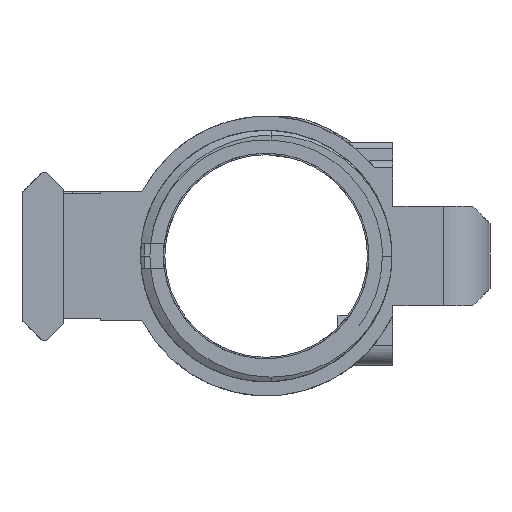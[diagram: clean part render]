
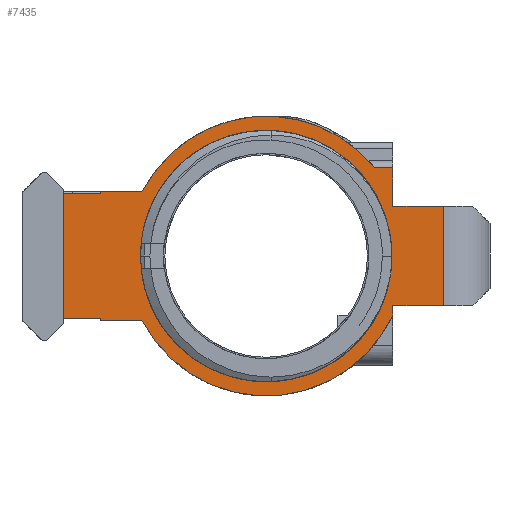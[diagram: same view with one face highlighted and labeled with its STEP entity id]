
A CAD part, left-side view. The second image highlights one B-rep face of the part: STEP entity #7435.
In plain terms, the highlighted planar face has unit normal (-1, 0, 0).
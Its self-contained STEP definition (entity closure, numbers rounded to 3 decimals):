
#105=FACE_BOUND('',#1064,.T.);
#117=CIRCLE('',#7738,17.621);
#195=CIRCLE('',#7919,17.621);
#202=CIRCLE('',#7934,14.891);
#347=PLANE('',#7933);
#659=FACE_OUTER_BOUND('',#1063,.T.);
#1063=EDGE_LOOP('',(#5813,#5814,#5815,#5816,#5817,#5818,#5819,#5820,#5821,
#5822,#5823,#5824,#5825,#5826,#5827,#5828,#5829,#5830,#5831));
#1064=EDGE_LOOP('',(#5832));
#1622=LINE('',#12179,#2366);
#1626=LINE('',#12186,#2370);
#1654=LINE('',#12771,#2398);
#1697=LINE('',#13081,#2441);
#1700=LINE('',#13086,#2444);
#1733=LINE('',#13286,#2477);
#1737=LINE('',#13296,#2481);
#1740=LINE('',#13302,#2484);
#1861=LINE('',#13553,#2605);
#1866=LINE('',#13570,#2610);
#1869=LINE('',#13587,#2613);
#1872=LINE('',#13595,#2616);
#1875=LINE('',#13603,#2619);
#1885=LINE('',#13627,#2629);
#1906=LINE('',#13778,#2650);
#1908=LINE('',#13787,#2652);
#1909=LINE('',#13788,#2653);
#2366=VECTOR('',#8499,10.);
#2370=VECTOR('',#8503,10.);
#2398=VECTOR('',#8599,10.);
#2441=VECTOR('',#8748,10.);
#2444=VECTOR('',#8753,10.);
#2477=VECTOR('',#8844,10.);
#2481=VECTOR('',#8852,10.);
#2484=VECTOR('',#8857,10.);
#2605=VECTOR('',#9000,10.);
#2610=VECTOR('',#9009,10.);
#2613=VECTOR('',#9014,10.);
#2616=VECTOR('',#9021,10.);
#2619=VECTOR('',#9028,10.);
#2629=VECTOR('',#9044,10.);
#2650=VECTOR('',#9091,10.);
#2652=VECTOR('',#9101,12.548);
#2653=VECTOR('',#9102,10.);
#3103=VERTEX_POINT('',#11544);
#3104=VERTEX_POINT('',#11546);
#3207=VERTEX_POINT('',#12176);
#3208=VERTEX_POINT('',#12178);
#3211=VERTEX_POINT('',#12184);
#3270=VERTEX_POINT('',#12770);
#3317=VERTEX_POINT('',#13077);
#3319=VERTEX_POINT('',#13080);
#3348=VERTEX_POINT('',#13276);
#3354=VERTEX_POINT('',#13289);
#3357=VERTEX_POINT('',#13298);
#3477=VERTEX_POINT('',#13552);
#3481=VERTEX_POINT('',#13567);
#3482=VERTEX_POINT('',#13572);
#3486=VERTEX_POINT('',#13590);
#3489=VERTEX_POINT('',#13598);
#3492=VERTEX_POINT('',#13606);
#3507=VERTEX_POINT('',#13682);
#3528=VERTEX_POINT('',#13777);
#3532=VERTEX_POINT('',#13789);
#3870=EDGE_CURVE('',#3103,#3104,#117,.T.);
#3995=EDGE_CURVE('',#3207,#3208,#1622,.T.);
#3999=EDGE_CURVE('',#3211,#3103,#1626,.T.);
#4072=EDGE_CURVE('',#3211,#3270,#1654,.F.);
#4157=EDGE_CURVE('',#3319,#3317,#1697,.T.);
#4160=EDGE_CURVE('',#3104,#3317,#1700,.T.);
#4213=EDGE_CURVE('',#3319,#3348,#1733,.T.);
#4218=EDGE_CURVE('',#3354,#3348,#1737,.T.);
#4221=EDGE_CURVE('',#3354,#3357,#1740,.T.);
#4347=EDGE_CURVE('',#3477,#3357,#1861,.T.);
#4354=EDGE_CURVE('',#3477,#3481,#1866,.T.);
#4358=EDGE_CURVE('',#3482,#3481,#1869,.T.);
#4362=EDGE_CURVE('',#3486,#3482,#1872,.T.);
#4366=EDGE_CURVE('',#3489,#3486,#1875,.T.);
#4378=EDGE_CURVE('',#3492,#3489,#1885,.F.);
#4385=EDGE_CURVE('',#3492,#3507,#195,.T.);
#4413=EDGE_CURVE('',#3528,#3208,#1906,.F.);
#4418=EDGE_CURVE('',#3270,#3528,#1908,.T.);
#4419=EDGE_CURVE('',#3207,#3507,#1909,.F.);
#4420=EDGE_CURVE('',#3532,#3532,#202,.T.);
#5813=ORIENTED_EDGE('',*,*,#4072,.T.);
#5814=ORIENTED_EDGE('',*,*,#4418,.T.);
#5815=ORIENTED_EDGE('',*,*,#4413,.T.);
#5816=ORIENTED_EDGE('',*,*,#3995,.F.);
#5817=ORIENTED_EDGE('',*,*,#4419,.T.);
#5818=ORIENTED_EDGE('',*,*,#4385,.F.);
#5819=ORIENTED_EDGE('',*,*,#4378,.T.);
#5820=ORIENTED_EDGE('',*,*,#4366,.T.);
#5821=ORIENTED_EDGE('',*,*,#4362,.T.);
#5822=ORIENTED_EDGE('',*,*,#4358,.T.);
#5823=ORIENTED_EDGE('',*,*,#4354,.F.);
#5824=ORIENTED_EDGE('',*,*,#4347,.T.);
#5825=ORIENTED_EDGE('',*,*,#4221,.F.);
#5826=ORIENTED_EDGE('',*,*,#4218,.T.);
#5827=ORIENTED_EDGE('',*,*,#4213,.F.);
#5828=ORIENTED_EDGE('',*,*,#4157,.T.);
#5829=ORIENTED_EDGE('',*,*,#4160,.F.);
#5830=ORIENTED_EDGE('',*,*,#3870,.F.);
#5831=ORIENTED_EDGE('',*,*,#3999,.F.);
#5832=ORIENTED_EDGE('',*,*,#4420,.T.);
#7435=ADVANCED_FACE('',(#659,#105),#347,.F.);
#7738=AXIS2_PLACEMENT_3D('',#11547,#8364,#8365);
#7919=AXIS2_PLACEMENT_3D('',#13683,#9050,#9051);
#7933=AXIS2_PLACEMENT_3D('',#13786,#9099,#9100);
#7934=AXIS2_PLACEMENT_3D('',#13790,#9103,#9104);
#8364=DIRECTION('center_axis',(1.,0.,0.));
#8365=DIRECTION('ref_axis',(0.,0.,-1.));
#8499=DIRECTION('',(0.,0.,-1.));
#8503=DIRECTION('',(0.,0.,-1.));
#8599=DIRECTION('',(0.,1.,0.));
#8748=DIRECTION('',(0.,0.,-1.));
#8753=DIRECTION('',(0.,1.,0.));
#8844=DIRECTION('',(0.,1.,0.));
#8852=DIRECTION('',(0.,0.,1.));
#8857=DIRECTION('',(0.,1.,0.));
#9000=DIRECTION('',(0.,0.,-1.));
#9009=DIRECTION('',(0.,-1.,0.));
#9014=DIRECTION('',(0.,0.,1.));
#9021=DIRECTION('',(0.,1.,0.));
#9028=DIRECTION('',(0.,0.,-1.));
#9044=DIRECTION('',(0.,-1.,0.));
#9050=DIRECTION('center_axis',(1.,0.,0.));
#9051=DIRECTION('ref_axis',(0.,0.,1.));
#9091=DIRECTION('',(0.,-1.,0.));
#9099=DIRECTION('center_axis',(1.,0.,0.));
#9100=DIRECTION('ref_axis',(0.,0.,-1.));
#9101=DIRECTION('',(0.,0.,1.));
#9102=DIRECTION('',(0.,-1.,0.));
#9103=DIRECTION('center_axis',(1.,0.,0.));
#9104=DIRECTION('ref_axis',(0.,0.,1.));
#11544=CARTESIAN_POINT('',(393.794,168.042,6.355));
#11546=CARTESIAN_POINT('',(393.794,199.673,5.699));
#11547=CARTESIAN_POINT('Origin',(393.794,184.018,13.789));
#12176=CARTESIAN_POINT('',(393.794,168.042,24.901));
#12178=CARTESIAN_POINT('',(393.794,168.042,20.063));
#12179=CARTESIAN_POINT('',(393.794,168.042,-1.067));
#12184=CARTESIAN_POINT('',(393.794,168.042,7.515));
#12186=CARTESIAN_POINT('',(393.794,168.042,-1.067));
#12770=CARTESIAN_POINT('',(393.794,161.692,7.515));
#12771=CARTESIAN_POINT('',(393.794,159.838,7.515));
#13077=CARTESIAN_POINT('',(393.794,204.872,5.699));
#13080=CARTESIAN_POINT('',(393.794,204.872,5.953));
#13081=CARTESIAN_POINT('',(393.794,204.872,2.159));
#13086=CARTESIAN_POINT('',(393.794,180.139,5.699));
#13276=CARTESIAN_POINT('',(393.794,209.571,5.953));
#13286=CARTESIAN_POINT('',(393.794,183.282,5.953));
#13289=CARTESIAN_POINT('',(393.794,209.571,5.699));
#13296=CARTESIAN_POINT('',(393.794,209.571,1.848));
#13298=CARTESIAN_POINT('',(393.794,209.594,5.699));
#13302=CARTESIAN_POINT('',(393.794,179.808,5.699));
#13552=CARTESIAN_POINT('',(393.794,209.594,21.879));
#13553=CARTESIAN_POINT('',(393.794,209.594,1.816));
#13567=CARTESIAN_POINT('',(393.794,209.571,21.879));
#13570=CARTESIAN_POINT('',(393.794,180.139,21.879));
#13572=CARTESIAN_POINT('',(393.794,209.571,21.625));
#13587=CARTESIAN_POINT('',(393.794,209.571,9.995));
#13590=CARTESIAN_POINT('',(393.794,204.872,21.625));
#13595=CARTESIAN_POINT('',(393.794,183.282,21.625));
#13598=CARTESIAN_POINT('',(393.794,204.872,21.879));
#13603=CARTESIAN_POINT('',(393.794,204.872,10.122));
#13606=CARTESIAN_POINT('',(393.794,199.673,21.879));
#13627=CARTESIAN_POINT('',(393.794,183.282,21.879));
#13682=CARTESIAN_POINT('',(393.794,170.343,24.901));
#13683=CARTESIAN_POINT('Origin',(393.794,184.018,13.789));
#13777=CARTESIAN_POINT('',(393.794,161.692,20.063));
#13778=CARTESIAN_POINT('',(393.794,164.867,20.063));
#13786=CARTESIAN_POINT('Origin',(393.794,161.692,-1.635));
#13787=CARTESIAN_POINT('',(393.794,161.692,7.515));
#13788=CARTESIAN_POINT('',(393.794,167.276,24.901));
#13789=CARTESIAN_POINT('',(393.794,184.018,-1.102));
#13790=CARTESIAN_POINT('Origin',(393.794,184.018,13.789));
